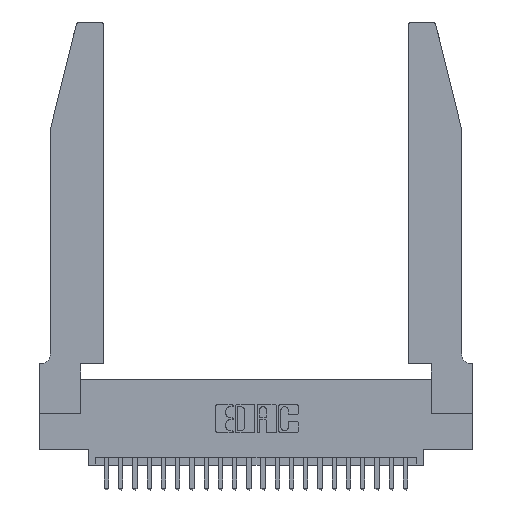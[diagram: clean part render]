
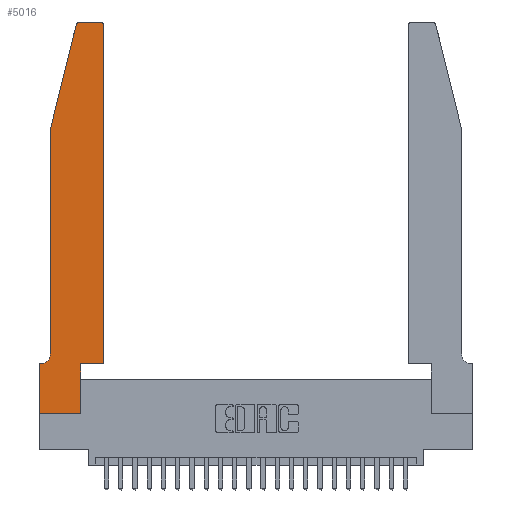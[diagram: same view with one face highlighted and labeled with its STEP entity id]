
A CAD part, top view. The second image highlights one B-rep face of the part: STEP entity #5016.
In plain terms, the highlighted planar face has unit normal (0, 0, 1).
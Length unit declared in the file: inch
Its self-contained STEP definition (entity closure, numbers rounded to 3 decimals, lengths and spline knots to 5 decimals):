
#8 = EDGE_CURVE ( 'NONE', #2894, #1533, #2826, .T. ) ;
#78 = DIRECTION ( 'NONE',  ( 1., 0., 0. ) ) ;
#172 = DIRECTION ( 'NONE',  ( 0., 1., 0. ) ) ;
#256 = CARTESIAN_POINT ( 'NONE',  ( 0.4205, 2.75, 0.37 ) ) ;
#285 = CARTESIAN_POINT ( 'NONE',  ( 0.4505, 0.35, 0.37 ) ) ;
#359 = CIRCLE ( 'NONE', #9101, 0.03 ) ;
#411 = ORIENTED_EDGE ( 'NONE', *, *, #1132, .T. ) ;
#550 = ORIENTED_EDGE ( 'NONE', *, *, #14626, .T. ) ;
#798 = VERTEX_POINT ( 'NONE', #6987 ) ;
#803 = ORIENTED_EDGE ( 'NONE', *, *, #10098, .T. ) ;
#812 = CARTESIAN_POINT ( 'NONE',  ( 0., 0., 0.37 ) ) ;
#824 = VECTOR ( 'NONE', #15952, 39.37008 ) ;
#1028 = EDGE_CURVE ( 'NONE', #14175, #2894, #2776, .T. ) ;
#1132 = EDGE_CURVE ( 'NONE', #798, #8602, #5488, .T. ) ;
#1387 = DIRECTION ( 'NONE',  ( 1., 0., 0. ) ) ;
#1533 = VERTEX_POINT ( 'NONE', #256 ) ;
#1935 = CARTESIAN_POINT ( 'NONE',  ( 0.0755, 2., 0.37 ) ) ;
#1938 = VERTEX_POINT ( 'NONE', #12658 ) ;
#2776 = LINE ( 'NONE', #8959, #3374 ) ;
#2826 = CIRCLE ( 'NONE', #23780, 0.03 ) ;
#2894 = VERTEX_POINT ( 'NONE', #23371 ) ;
#3323 = CARTESIAN_POINT ( 'NONE',  ( 0.0055, 0.42, 0.37 ) ) ;
#3374 = VECTOR ( 'NONE', #12301, 39.37008 ) ;
#3398 = DIRECTION ( 'NONE',  ( 0., 0., -1. ) ) ;
#3565 = DIRECTION ( 'NONE',  ( 0., 0., 1. ) ) ;
#4011 = CARTESIAN_POINT ( 'NONE',  ( 0.2605, 2.75, 0.37 ) ) ;
#4052 = ORIENTED_EDGE ( 'NONE', *, *, #19194, .T. ) ;
#4370 = VECTOR ( 'NONE', #15707, 39.37008 ) ;
#5016 = ADVANCED_FACE ( 'NONE', ( #15818 ), #5816, .T. ) ;
#5026 = CARTESIAN_POINT ( 'NONE',  ( 0.4205, 2.72, 0.37 ) ) ;
#5075 = VECTOR ( 'NONE', #8179, 39.37008 ) ;
#5108 = ORIENTED_EDGE ( 'NONE', *, *, #1028, .T. ) ;
#5488 = CIRCLE ( 'NONE', #24442, 0.07 ) ;
#5540 = VECTOR ( 'NONE', #15522, 39.37008 ) ;
#5544 = CARTESIAN_POINT ( 'NONE',  ( 0.2865, 0., 0.37 ) ) ;
#5687 = VERTEX_POINT ( 'NONE', #5871 ) ;
#5816 = PLANE ( 'NONE',  #16104 ) ;
#5871 = CARTESIAN_POINT ( 'NONE',  ( 0.284, 2.75, 0.37 ) ) ;
#6055 = ORIENTED_EDGE ( 'NONE', *, *, #13611, .T. ) ;
#6245 = CARTESIAN_POINT ( 'NONE',  ( 0.0755, 2., 0.37 ) ) ;
#6971 = DIRECTION ( 'NONE',  ( 1., 0., 0. ) ) ;
#6987 = CARTESIAN_POINT ( 'NONE',  ( 0.0755, 0.42, 0.37 ) ) ;
#7363 = VERTEX_POINT ( 'NONE', #5544 ) ;
#7518 = DIRECTION ( 'NONE',  ( -1., 0., 0. ) ) ;
#7555 = CARTESIAN_POINT ( 'NONE',  ( 0.4505, 0.35, 0.37 ) ) ;
#7684 = EDGE_CURVE ( 'NONE', #8699, #19764, #9041, .T. ) ;
#7883 = DIRECTION ( 'NONE',  ( -1., 0., 0. ) ) ;
#8179 = DIRECTION ( 'NONE',  ( -0.239, -0.971, 0. ) ) ;
#8406 = ORIENTED_EDGE ( 'NONE', *, *, #17702, .T. ) ;
#8602 = VERTEX_POINT ( 'NONE', #11310 ) ;
#8699 = VERTEX_POINT ( 'NONE', #11890 ) ;
#8784 = CARTESIAN_POINT ( 'NONE',  ( 0., 0., 0.37 ) ) ;
#8959 = CARTESIAN_POINT ( 'NONE',  ( 0.4505, 0.35, 0.37 ) ) ;
#9041 = LINE ( 'NONE', #812, #18091 ) ;
#9101 = AXIS2_PLACEMENT_3D ( 'NONE', #22339, #10802, #24285 ) ;
#9674 = VECTOR ( 'NONE', #7883, 39.37008 ) ;
#10027 = ORIENTED_EDGE ( 'NONE', *, *, #13647, .T. ) ;
#10098 = EDGE_CURVE ( 'NONE', #12896, #10252, #15327, .T. ) ;
#10252 = VERTEX_POINT ( 'NONE', #24037 ) ;
#10685 = LINE ( 'NONE', #23255, #24822 ) ;
#10802 = DIRECTION ( 'NONE',  ( 0., 0., 1. ) ) ;
#11310 = CARTESIAN_POINT ( 'NONE',  ( 0.0055, 0.35, 0.37 ) ) ;
#11641 = DIRECTION ( 'NONE',  ( 0., 0., 1. ) ) ;
#11890 = CARTESIAN_POINT ( 'NONE',  ( 0., 0.35, 0.37 ) ) ;
#12301 = DIRECTION ( 'NONE',  ( 0., 1., 0. ) ) ;
#12658 = CARTESIAN_POINT ( 'NONE',  ( 0.2865, 0.35, 0.37 ) ) ;
#12896 = VERTEX_POINT ( 'NONE', #18208 ) ;
#13100 = LINE ( 'NONE', #18505, #23331 ) ;
#13611 = EDGE_CURVE ( 'NONE', #10252, #798, #15797, .T. ) ;
#13614 = EDGE_LOOP ( 'NONE', ( #17365, #550, #803, #6055, #411, #14494, #16151, #4052, #10027, #8406, #5108, #17344 ) ) ;
#13647 = EDGE_CURVE ( 'NONE', #7363, #1938, #10685, .T. ) ;
#14175 = VERTEX_POINT ( 'NONE', #7555 ) ;
#14494 = ORIENTED_EDGE ( 'NONE', *, *, #16535, .T. ) ;
#14626 = EDGE_CURVE ( 'NONE', #5687, #12896, #359, .T. ) ;
#15327 = LINE ( 'NONE', #6245, #5075 ) ;
#15438 = LINE ( 'NONE', #4011, #9674 ) ;
#15522 = DIRECTION ( 'NONE',  ( 0., -1., 0. ) ) ;
#15707 = DIRECTION ( 'NONE',  ( 1., 0., 0. ) ) ;
#15797 = LINE ( 'NONE', #1935, #5540 ) ;
#15818 = FACE_OUTER_BOUND ( 'NONE', #13614, .T. ) ;
#15952 = DIRECTION ( 'NONE',  ( -1., 0., 0. ) ) ;
#16104 = AXIS2_PLACEMENT_3D ( 'NONE', #19283, #11641, #78 ) ;
#16151 = ORIENTED_EDGE ( 'NONE', *, *, #7684, .T. ) ;
#16535 = EDGE_CURVE ( 'NONE', #8602, #8699, #20720, .T. ) ;
#17344 = ORIENTED_EDGE ( 'NONE', *, *, #8, .T. ) ;
#17365 = ORIENTED_EDGE ( 'NONE', *, *, #23841, .T. ) ;
#17702 = EDGE_CURVE ( 'NONE', #1938, #14175, #24873, .T. ) ;
#18079 = DIRECTION ( 'NONE',  ( 0., -1., 0. ) ) ;
#18091 = VECTOR ( 'NONE', #18079, 39.37008 ) ;
#18208 = CARTESIAN_POINT ( 'NONE',  ( 0.25487, 2.72718, 0.37 ) ) ;
#18505 = CARTESIAN_POINT ( 'NONE',  ( 0., 0., 0.37 ) ) ;
#19194 = EDGE_CURVE ( 'NONE', #19764, #7363, #13100, .T. ) ;
#19283 = CARTESIAN_POINT ( 'NONE',  ( 0., 0.35, 0.37 ) ) ;
#19764 = VERTEX_POINT ( 'NONE', #8784 ) ;
#20720 = LINE ( 'NONE', #23702, #824 ) ;
#22339 = CARTESIAN_POINT ( 'NONE',  ( 0.284, 2.72, 0.37 ) ) ;
#23255 = CARTESIAN_POINT ( 'NONE',  ( 0.2865, 0.35, 0.37 ) ) ;
#23331 = VECTOR ( 'NONE', #6971, 39.37008 ) ;
#23371 = CARTESIAN_POINT ( 'NONE',  ( 0.4505, 2.72, 0.37 ) ) ;
#23702 = CARTESIAN_POINT ( 'NONE',  ( 0.0755, 0.35, 0.37 ) ) ;
#23780 = AXIS2_PLACEMENT_3D ( 'NONE', #5026, #3565, #1387 ) ;
#23841 = EDGE_CURVE ( 'NONE', #1533, #5687, #15438, .T. ) ;
#24037 = CARTESIAN_POINT ( 'NONE',  ( 0.0755, 2., 0.37 ) ) ;
#24285 = DIRECTION ( 'NONE',  ( 1., 0., 0. ) ) ;
#24442 = AXIS2_PLACEMENT_3D ( 'NONE', #3323, #3398, #7518 ) ;
#24822 = VECTOR ( 'NONE', #172, 39.37008 ) ;
#24873 = LINE ( 'NONE', #285, #4370 ) ;
